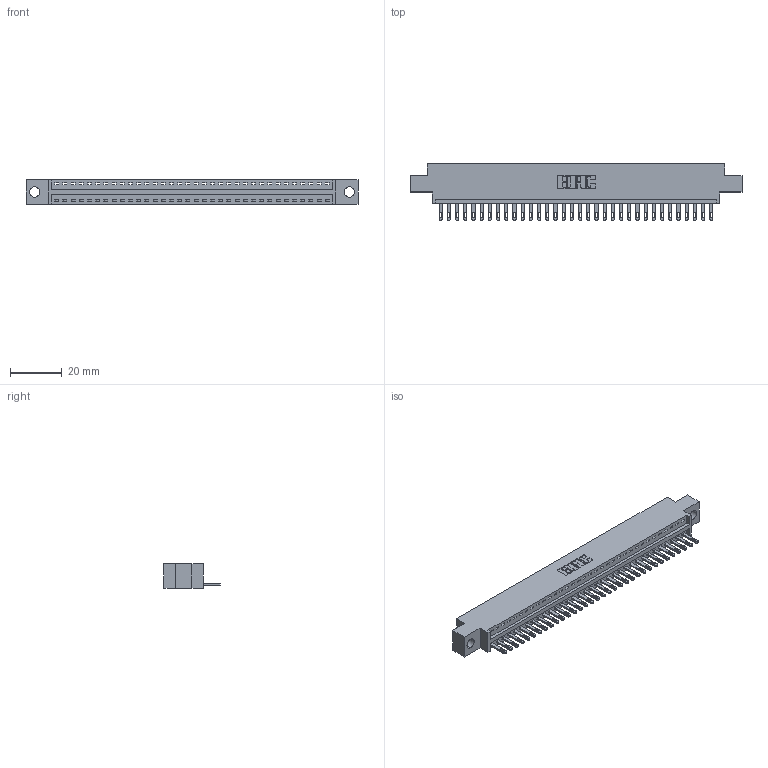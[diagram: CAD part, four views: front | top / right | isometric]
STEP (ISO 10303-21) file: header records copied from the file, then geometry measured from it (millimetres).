
FILE_DESCRIPTION (( 'STEP AP203' ), '1' );
FILE_NAME ('346-034-500-604.STEP', '2018-08-23T21:34:14', ( '' ), ( '' ), 'SwSTEP 2.0', 'SolidWorks 2016', '' );
FILE_SCHEMA (( 'CONFIG_CONTROL_DESIGN' ));
Length unit declared in the file: inch
Products named in the file (3): 345-292-001_345-293-100; 346-034-500-604; 346 Part_0.170 Offset - 0.156 Dia-TH
Assembly tree (35 placements, depth 2):
  346-034-500-604
    346 Part_0.170 Offset - 0.156 Dia-TH
    345-292-001_345-293-100  x34
Bounding box: 128.52 x 21.84 x 9.4 mm (x, y, z)
Volume: 12026 mm3; surface area: 14989.2 mm2
Topology: 35 solids, 35 shells, 1962 faces, 6053 edges, 4034 vertices
Faces by surface type: plane 1236, cylinder 726
Entity records: 22243 total; most frequent: CARTESIAN_POINT 3822, ORIENTED_EDGE 3790, DIRECTION 3383, EDGE_CURVE 1895, VECTOR 1623, LINE 1623, VERTEX_POINT 1262, AXIS2_PLACEMENT_3D 880
